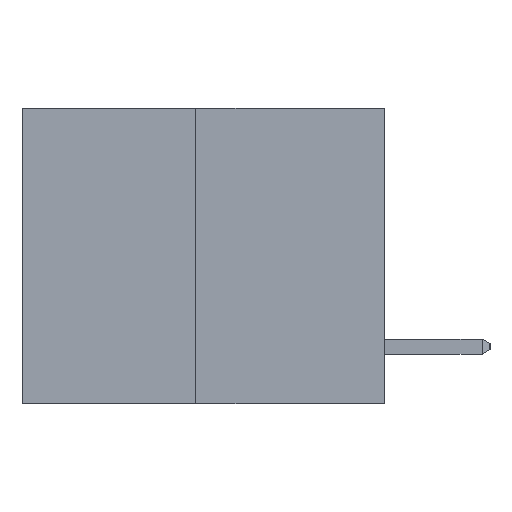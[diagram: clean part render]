
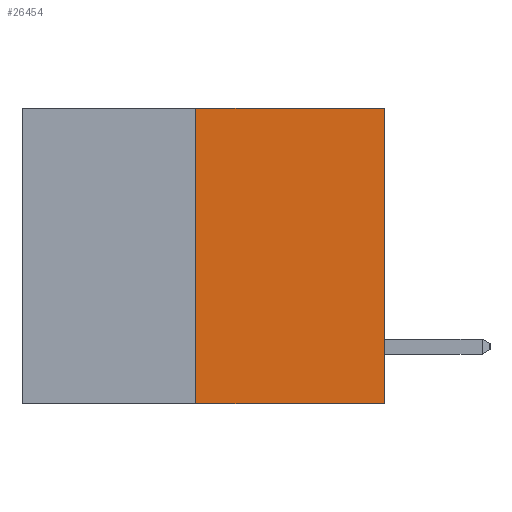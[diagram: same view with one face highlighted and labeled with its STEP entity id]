
A CAD part, left-side view. The second image highlights one B-rep face of the part: STEP entity #26454.
In plain terms, the highlighted planar face has unit normal (-1, 0, 0).
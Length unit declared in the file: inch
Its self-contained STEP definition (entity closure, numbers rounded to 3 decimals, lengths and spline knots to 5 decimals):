
#633 = VERTEX_POINT ( 'NONE', #13822 ) ;
#675 = VECTOR ( 'NONE', #21910, 39.37008 ) ;
#2840 = LINE ( 'NONE', #11491, #10383 ) ;
#3131 = LINE ( 'NONE', #17560, #6015 ) ;
#3808 = DIRECTION ( 'NONE',  ( 0., -1., 0. ) ) ;
#4905 = VERTEX_POINT ( 'NONE', #5244 ) ;
#5244 = CARTESIAN_POINT ( 'NONE',  ( 0., 0.312, -0.49 ) ) ;
#6015 = VECTOR ( 'NONE', #3808, 39.37008 ) ;
#6049 = CARTESIAN_POINT ( 'NONE',  ( 0., 0.6, 0. ) ) ;
#10247 = ORIENTED_EDGE ( 'NONE', *, *, #19996, .T. ) ;
#10383 = VECTOR ( 'NONE', #27591, 39.37008 ) ;
#10576 = PLANE ( 'NONE',  #20869 ) ;
#11256 = EDGE_LOOP ( 'NONE', ( #15211, #10247, #25369, #18712 ) ) ;
#11491 = CARTESIAN_POINT ( 'NONE',  ( 0., 0.312, -0.49 ) ) ;
#13138 = VERTEX_POINT ( 'NONE', #23831 ) ;
#13822 = CARTESIAN_POINT ( 'NONE',  ( 0., 0., -0.49 ) ) ;
#14450 = EDGE_CURVE ( 'NONE', #13138, #18368, #16158, .T. ) ;
#14678 = EDGE_CURVE ( 'NONE', #4905, #13138, #2840, .T. ) ;
#15211 = ORIENTED_EDGE ( 'NONE', *, *, #14678, .F. ) ;
#15302 = CARTESIAN_POINT ( 'NONE',  ( 0., 0., 0. ) ) ;
#16158 = LINE ( 'NONE', #23863, #16511 ) ;
#16511 = VECTOR ( 'NONE', #19344, 39.37008 ) ;
#17560 = CARTESIAN_POINT ( 'NONE',  ( 0., 0.6, -0.49 ) ) ;
#18368 = VERTEX_POINT ( 'NONE', #27174 ) ;
#18712 = ORIENTED_EDGE ( 'NONE', *, *, #14450, .F. ) ;
#19344 = DIRECTION ( 'NONE',  ( 0., -1., 0. ) ) ;
#19996 = EDGE_CURVE ( 'NONE', #4905, #633, #3131, .T. ) ;
#20022 = DIRECTION ( 'NONE',  ( 1., 0., 0. ) ) ;
#20161 = FACE_OUTER_BOUND ( 'NONE', #11256, .T. ) ;
#20869 = AXIS2_PLACEMENT_3D ( 'NONE', #6049, #20022, #22213 ) ;
#21910 = DIRECTION ( 'NONE',  ( 0., 0., 1. ) ) ;
#22213 = DIRECTION ( 'NONE',  ( 0., 0., -1. ) ) ;
#23316 = LINE ( 'NONE', #15302, #675 ) ;
#23831 = CARTESIAN_POINT ( 'NONE',  ( 0., 0.312, 0. ) ) ;
#23863 = CARTESIAN_POINT ( 'NONE',  ( 0., 0.6, 0. ) ) ;
#25369 = ORIENTED_EDGE ( 'NONE', *, *, #27239, .T. ) ;
#26454 = ADVANCED_FACE ( 'NONE', ( #20161 ), #10576, .F. ) ;
#27174 = CARTESIAN_POINT ( 'NONE',  ( 0., 0., 0. ) ) ;
#27239 = EDGE_CURVE ( 'NONE', #633, #18368, #23316, .T. ) ;
#27591 = DIRECTION ( 'NONE',  ( 0., 0., 1. ) ) ;
